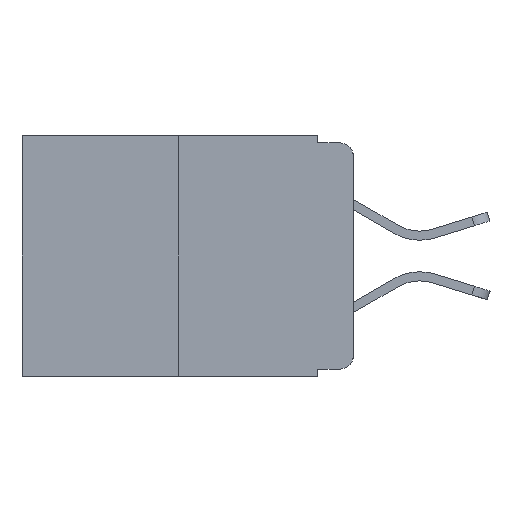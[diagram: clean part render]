
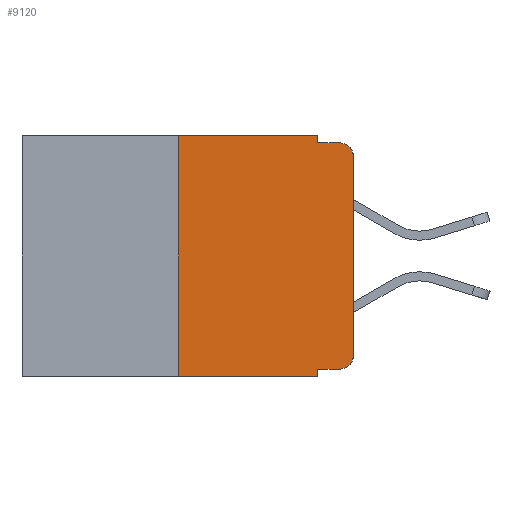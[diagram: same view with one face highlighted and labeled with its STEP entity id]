
A CAD part, left-side view. The second image highlights one B-rep face of the part: STEP entity #9120.
In plain terms, the highlighted planar face has unit normal (-1, 0, 0).
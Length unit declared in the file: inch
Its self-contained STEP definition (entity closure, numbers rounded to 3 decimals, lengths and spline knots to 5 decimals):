
#56 = VERTEX_POINT ( 'NONE', #1507 ) ;
#225 = LINE ( 'NONE', #5626, #3079 ) ;
#638 = ORIENTED_EDGE ( 'NONE', *, *, #4609, .T. ) ;
#787 = CARTESIAN_POINT ( 'NONE',  ( 0., 0.02, -0.03 ) ) ;
#882 = LINE ( 'NONE', #2205, #9364 ) ;
#918 = DIRECTION ( 'NONE',  ( 1., 0., 0. ) ) ;
#959 = ORIENTED_EDGE ( 'NONE', *, *, #1203, .T. ) ;
#1202 = EDGE_CURVE ( 'NONE', #4015, #2586, #8251, .T. ) ;
#1203 = EDGE_CURVE ( 'NONE', #4015, #2864, #4321, .T. ) ;
#1496 = CARTESIAN_POINT ( 'NONE',  ( 0., 0.051, -0.01 ) ) ;
#1507 = CARTESIAN_POINT ( 'NONE',  ( 0., 0.25, -0.343 ) ) ;
#1781 = CIRCLE ( 'NONE', #3235, 0.02 ) ;
#1949 = CARTESIAN_POINT ( 'NONE',  ( 0., 0.051, -0.333 ) ) ;
#1981 = LINE ( 'NONE', #5833, #8636 ) ;
#2088 = DIRECTION ( 'NONE',  ( 0., 0., -1. ) ) ;
#2205 = CARTESIAN_POINT ( 'NONE',  ( 0., 0.473, -0.343 ) ) ;
#2258 = VECTOR ( 'NONE', #5313, 39.37008 ) ;
#2269 = CARTESIAN_POINT ( 'NONE',  ( 0., 0.051, 0. ) ) ;
#2321 = CARTESIAN_POINT ( 'NONE',  ( 0., 0.02, -0.333 ) ) ;
#2436 = EDGE_CURVE ( 'NONE', #2864, #6115, #1781, .T. ) ;
#2578 = EDGE_CURVE ( 'NONE', #56, #3041, #225, .T. ) ;
#2586 = VERTEX_POINT ( 'NONE', #4174 ) ;
#2695 = ORIENTED_EDGE ( 'NONE', *, *, #1202, .F. ) ;
#2758 = CARTESIAN_POINT ( 'NONE',  ( 0., 0.051, -0.01 ) ) ;
#2821 = CARTESIAN_POINT ( 'NONE',  ( 0., 0.02, -0.01 ) ) ;
#2864 = VERTEX_POINT ( 'NONE', #2321 ) ;
#3025 = AXIS2_PLACEMENT_3D ( 'NONE', #3297, #918, #4092 ) ;
#3041 = VERTEX_POINT ( 'NONE', #4462 ) ;
#3079 = VECTOR ( 'NONE', #6390, 39.37008 ) ;
#3235 = AXIS2_PLACEMENT_3D ( 'NONE', #7230, #8094, #9518 ) ;
#3289 = ORIENTED_EDGE ( 'NONE', *, *, #4824, .F. ) ;
#3297 = CARTESIAN_POINT ( 'NONE',  ( 0., 0.473, 0. ) ) ;
#3512 = EDGE_LOOP ( 'NONE', ( #8638, #638, #3289, #4123, #7265, #5680, #3612, #2695, #959, #5578 ) ) ;
#3612 = ORIENTED_EDGE ( 'NONE', *, *, #7765, .T. ) ;
#3634 = CARTESIAN_POINT ( 'NONE',  ( 0., 0., -0.313 ) ) ;
#3760 = DIRECTION ( 'NONE',  ( 0., 0., -1. ) ) ;
#3903 = DIRECTION ( 'NONE',  ( -1., 0., 0. ) ) ;
#3981 = PLANE ( 'NONE',  #3025 ) ;
#4015 = VERTEX_POINT ( 'NONE', #1949 ) ;
#4047 = VECTOR ( 'NONE', #4126, 39.37008 ) ;
#4049 = VECTOR ( 'NONE', #2088, 39.37008 ) ;
#4092 = DIRECTION ( 'NONE',  ( 0., 0., -1. ) ) ;
#4123 = ORIENTED_EDGE ( 'NONE', *, *, #5558, .F. ) ;
#4126 = DIRECTION ( 'NONE',  ( 0., 0., 1. ) ) ;
#4174 = CARTESIAN_POINT ( 'NONE',  ( 0., 0.051, -0.343 ) ) ;
#4250 = LINE ( 'NONE', #2758, #4390 ) ;
#4286 = LINE ( 'NONE', #5090, #4049 ) ;
#4321 = LINE ( 'NONE', #5925, #7867 ) ;
#4390 = VECTOR ( 'NONE', #5956, 39.37008 ) ;
#4462 = CARTESIAN_POINT ( 'NONE',  ( 0., 0.25, 0. ) ) ;
#4554 = VERTEX_POINT ( 'NONE', #2821 ) ;
#4609 = EDGE_CURVE ( 'NONE', #8263, #4554, #4977, .T. ) ;
#4824 = EDGE_CURVE ( 'NONE', #8640, #4554, #4250, .T. ) ;
#4977 = CIRCLE ( 'NONE', #6270, 0.02 ) ;
#5090 = CARTESIAN_POINT ( 'NONE',  ( 0., 0.051, 0. ) ) ;
#5173 = DIRECTION ( 'NONE',  ( 0., -1., 0. ) ) ;
#5313 = DIRECTION ( 'NONE',  ( 0., 0., -1. ) ) ;
#5347 = DIRECTION ( 'NONE',  ( 0., -1., 0. ) ) ;
#5545 = FACE_OUTER_BOUND ( 'NONE', #3512, .T. ) ;
#5558 = EDGE_CURVE ( 'NONE', #6936, #8640, #4286, .T. ) ;
#5578 = ORIENTED_EDGE ( 'NONE', *, *, #2436, .T. ) ;
#5626 = CARTESIAN_POINT ( 'NONE',  ( 0., 0.25, 0. ) ) ;
#5680 = ORIENTED_EDGE ( 'NONE', *, *, #2578, .F. ) ;
#5833 = CARTESIAN_POINT ( 'NONE',  ( 0., 0.473, 0. ) ) ;
#5925 = CARTESIAN_POINT ( 'NONE',  ( 0., 0.051, -0.333 ) ) ;
#5956 = DIRECTION ( 'NONE',  ( 0., -1., 0. ) ) ;
#6115 = VERTEX_POINT ( 'NONE', #3634 ) ;
#6270 = AXIS2_PLACEMENT_3D ( 'NONE', #787, #3903, #3760 ) ;
#6390 = DIRECTION ( 'NONE',  ( 0., 0., 1. ) ) ;
#6655 = LINE ( 'NONE', #9702, #4047 ) ;
#6862 = CARTESIAN_POINT ( 'NONE',  ( 0., 0., -0.03 ) ) ;
#6936 = VERTEX_POINT ( 'NONE', #7481 ) ;
#7064 = EDGE_CURVE ( 'NONE', #6115, #8263, #6655, .T. ) ;
#7230 = CARTESIAN_POINT ( 'NONE',  ( 0., 0.02, -0.313 ) ) ;
#7265 = ORIENTED_EDGE ( 'NONE', *, *, #9643, .F. ) ;
#7481 = CARTESIAN_POINT ( 'NONE',  ( 0., 0.051, 0. ) ) ;
#7765 = EDGE_CURVE ( 'NONE', #56, #2586, #882, .T. ) ;
#7867 = VECTOR ( 'NONE', #5173, 39.37008 ) ;
#8094 = DIRECTION ( 'NONE',  ( -1., 0., 0. ) ) ;
#8251 = LINE ( 'NONE', #2269, #2258 ) ;
#8263 = VERTEX_POINT ( 'NONE', #6862 ) ;
#8636 = VECTOR ( 'NONE', #9692, 39.37008 ) ;
#8638 = ORIENTED_EDGE ( 'NONE', *, *, #7064, .T. ) ;
#8640 = VERTEX_POINT ( 'NONE', #1496 ) ;
#9120 = ADVANCED_FACE ( 'NONE', ( #5545 ), #3981, .F. ) ;
#9364 = VECTOR ( 'NONE', #5347, 39.37008 ) ;
#9518 = DIRECTION ( 'NONE',  ( 0., 0., -1. ) ) ;
#9643 = EDGE_CURVE ( 'NONE', #3041, #6936, #1981, .T. ) ;
#9692 = DIRECTION ( 'NONE',  ( 0., -1., 0. ) ) ;
#9702 = CARTESIAN_POINT ( 'NONE',  ( 0., 0., 0. ) ) ;
